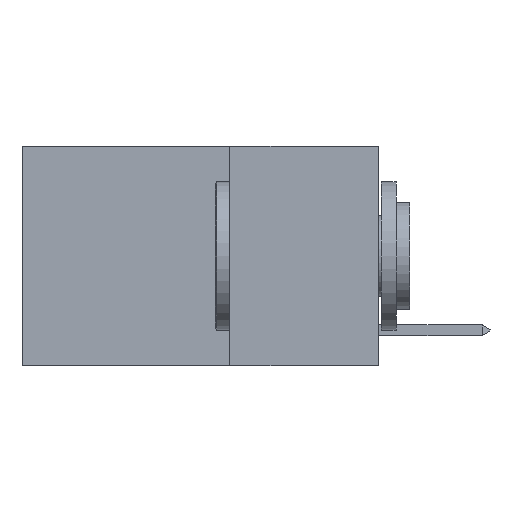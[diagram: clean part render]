
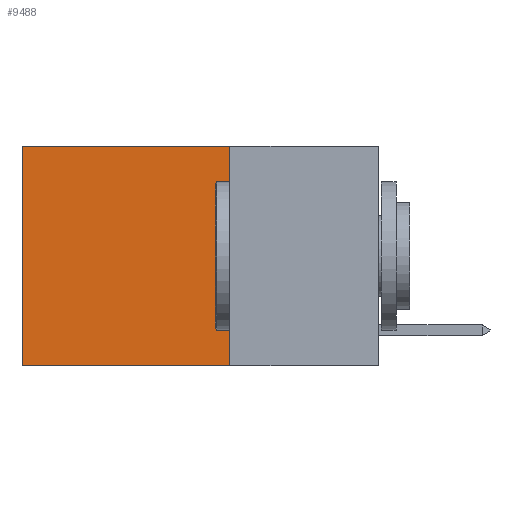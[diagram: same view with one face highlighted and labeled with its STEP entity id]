
A CAD part, left-side view. The second image highlights one B-rep face of the part: STEP entity #9488.
In plain terms, the highlighted planar face has unit normal (-1, 0, 0).
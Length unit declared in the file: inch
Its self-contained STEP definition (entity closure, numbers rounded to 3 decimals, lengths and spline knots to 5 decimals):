
#917 = VECTOR ( 'NONE', #11017, 39.37008 ) ;
#1019 = CARTESIAN_POINT ( 'NONE',  ( 0.2625, 0.6, -0.37 ) ) ;
#1677 = ORIENTED_EDGE ( 'NONE', *, *, #16387, .T. ) ;
#1991 = PLANE ( 'NONE',  #18778 ) ;
#2166 = ORIENTED_EDGE ( 'NONE', *, *, #6903, .F. ) ;
#2932 = CARTESIAN_POINT ( 'NONE',  ( 0.2625, 0.25, -0.37 ) ) ;
#4143 = VECTOR ( 'NONE', #13056, 39.37008 ) ;
#4590 = FACE_OUTER_BOUND ( 'NONE', #14646, .T. ) ;
#5123 = CARTESIAN_POINT ( 'NONE',  ( 0.2625, 0.25, -0.37 ) ) ;
#5143 = LINE ( 'NONE', #10302, #13885 ) ;
#5273 = LINE ( 'NONE', #8473, #4143 ) ;
#6746 = VECTOR ( 'NONE', #17403, 39.37008 ) ;
#6903 = EDGE_CURVE ( 'NONE', #10419, #8398, #14980, .T. ) ;
#8305 = ORIENTED_EDGE ( 'NONE', *, *, #13351, .T. ) ;
#8398 = VERTEX_POINT ( 'NONE', #1019 ) ;
#8473 = CARTESIAN_POINT ( 'NONE',  ( 0.2625, 0.25, 0. ) ) ;
#9488 = ADVANCED_FACE ( 'NONE', ( #4590 ), #1991, .F. ) ;
#10108 = CARTESIAN_POINT ( 'NONE',  ( 0.2625, 0.25, 0. ) ) ;
#10302 = CARTESIAN_POINT ( 'NONE',  ( 0.2625, 0.6, 0. ) ) ;
#10382 = CARTESIAN_POINT ( 'NONE',  ( 0.2625, 0.6, 0. ) ) ;
#10419 = VERTEX_POINT ( 'NONE', #2932 ) ;
#11017 = DIRECTION ( 'NONE',  ( 0., 1., 0. ) ) ;
#12380 = VERTEX_POINT ( 'NONE', #14353 ) ;
#12408 = EDGE_CURVE ( 'NONE', #12380, #10419, #13002, .T. ) ;
#13002 = LINE ( 'NONE', #10108, #6746 ) ;
#13056 = DIRECTION ( 'NONE',  ( 0., 1., 0. ) ) ;
#13351 = EDGE_CURVE ( 'NONE', #18886, #8398, #5143, .T. ) ;
#13885 = VECTOR ( 'NONE', #14553, 39.37008 ) ;
#13960 = CARTESIAN_POINT ( 'NONE',  ( 0.2625, 0.25, 0. ) ) ;
#14353 = CARTESIAN_POINT ( 'NONE',  ( 0.2625, 0.25, 0. ) ) ;
#14553 = DIRECTION ( 'NONE',  ( 0., 0., -1. ) ) ;
#14646 = EDGE_LOOP ( 'NONE', ( #8305, #2166, #17938, #1677 ) ) ;
#14980 = LINE ( 'NONE', #5123, #917 ) ;
#15312 = DIRECTION ( 'NONE',  ( 1., 0., 0. ) ) ;
#16387 = EDGE_CURVE ( 'NONE', #12380, #18886, #5273, .T. ) ;
#17403 = DIRECTION ( 'NONE',  ( 0., 0., -1. ) ) ;
#17938 = ORIENTED_EDGE ( 'NONE', *, *, #12408, .F. ) ;
#18218 = DIRECTION ( 'NONE',  ( 0., 0., -1. ) ) ;
#18778 = AXIS2_PLACEMENT_3D ( 'NONE', #13960, #15312, #18218 ) ;
#18886 = VERTEX_POINT ( 'NONE', #10382 ) ;
